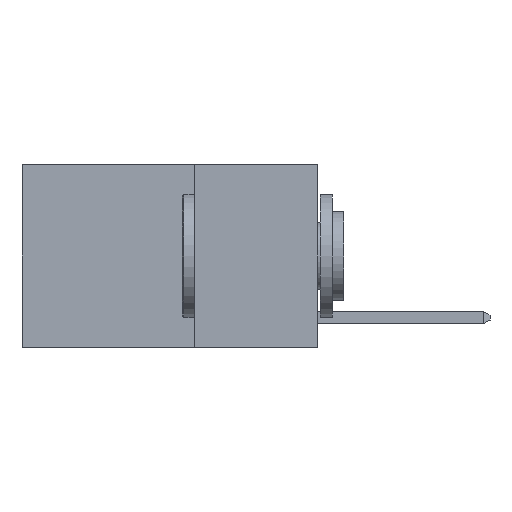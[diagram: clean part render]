
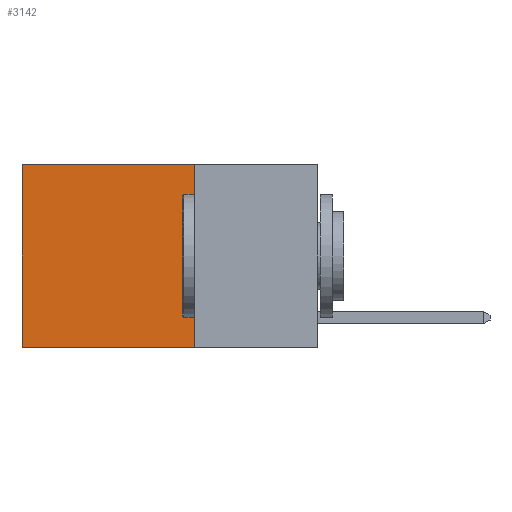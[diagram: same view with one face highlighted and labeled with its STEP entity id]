
A CAD part, left-side view. The second image highlights one B-rep face of the part: STEP entity #3142.
In plain terms, the highlighted planar face has unit normal (-1, 0, 0).
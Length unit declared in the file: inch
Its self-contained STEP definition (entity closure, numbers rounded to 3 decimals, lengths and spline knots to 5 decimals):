
#28 = CARTESIAN_POINT ( 'NONE',  ( 0.2625, 0.6, 0. ) ) ;
#38 = PLANE ( 'NONE',  #1455 ) ;
#635 = CARTESIAN_POINT ( 'NONE',  ( 0.2625, 0.25, 0. ) ) ;
#957 = DIRECTION ( 'NONE',  ( 1., 0., 0. ) ) ;
#972 = VERTEX_POINT ( 'NONE', #635 ) ;
#1235 = ORIENTED_EDGE ( 'NONE', *, *, #3540, .T. ) ;
#1455 = AXIS2_PLACEMENT_3D ( 'NONE', #6028, #957, #6834 ) ;
#2140 = ORIENTED_EDGE ( 'NONE', *, *, #3953, .F. ) ;
#2785 = VECTOR ( 'NONE', #10286, 39.37008 ) ;
#2786 = EDGE_CURVE ( 'NONE', #972, #3389, #5001, .T. ) ;
#3142 = ADVANCED_FACE ( 'NONE', ( #5501 ), #38, .F. ) ;
#3272 = VERTEX_POINT ( 'NONE', #9303 ) ;
#3389 = VERTEX_POINT ( 'NONE', #5640 ) ;
#3444 = DIRECTION ( 'NONE',  ( 0., 1., 0. ) ) ;
#3540 = EDGE_CURVE ( 'NONE', #3272, #7067, #8823, .T. ) ;
#3877 = ORIENTED_EDGE ( 'NONE', *, *, #2786, .F. ) ;
#3953 = EDGE_CURVE ( 'NONE', #3389, #7067, #5459, .T. ) ;
#4305 = LINE ( 'NONE', #9748, #8289 ) ;
#5001 = LINE ( 'NONE', #7114, #2785 ) ;
#5158 = ORIENTED_EDGE ( 'NONE', *, *, #5619, .T. ) ;
#5459 = LINE ( 'NONE', #8255, #9670 ) ;
#5501 = FACE_OUTER_BOUND ( 'NONE', #7697, .T. ) ;
#5619 = EDGE_CURVE ( 'NONE', #972, #3272, #4305, .T. ) ;
#5640 = CARTESIAN_POINT ( 'NONE',  ( 0.2625, 0.25, -0.37 ) ) ;
#5802 = DIRECTION ( 'NONE',  ( 0., 1., 0. ) ) ;
#6028 = CARTESIAN_POINT ( 'NONE',  ( 0.2625, 0.25, 0. ) ) ;
#6472 = VECTOR ( 'NONE', #7610, 39.37008 ) ;
#6543 = CARTESIAN_POINT ( 'NONE',  ( 0.2625, 0.6, -0.37 ) ) ;
#6834 = DIRECTION ( 'NONE',  ( 0., 0., -1. ) ) ;
#7067 = VERTEX_POINT ( 'NONE', #6543 ) ;
#7114 = CARTESIAN_POINT ( 'NONE',  ( 0.2625, 0.25, 0. ) ) ;
#7610 = DIRECTION ( 'NONE',  ( 0., 0., -1. ) ) ;
#7697 = EDGE_LOOP ( 'NONE', ( #1235, #2140, #3877, #5158 ) ) ;
#8255 = CARTESIAN_POINT ( 'NONE',  ( 0.2625, 0.25, -0.37 ) ) ;
#8289 = VECTOR ( 'NONE', #5802, 39.37008 ) ;
#8823 = LINE ( 'NONE', #28, #6472 ) ;
#9303 = CARTESIAN_POINT ( 'NONE',  ( 0.2625, 0.6, 0. ) ) ;
#9670 = VECTOR ( 'NONE', #3444, 39.37008 ) ;
#9748 = CARTESIAN_POINT ( 'NONE',  ( 0.2625, 0.25, 0. ) ) ;
#10286 = DIRECTION ( 'NONE',  ( 0., 0., -1. ) ) ;
